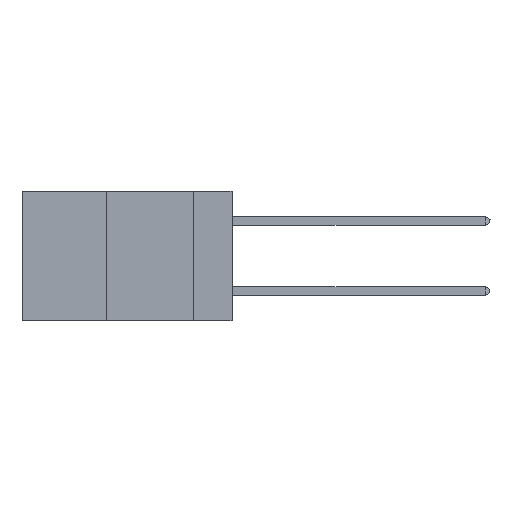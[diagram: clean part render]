
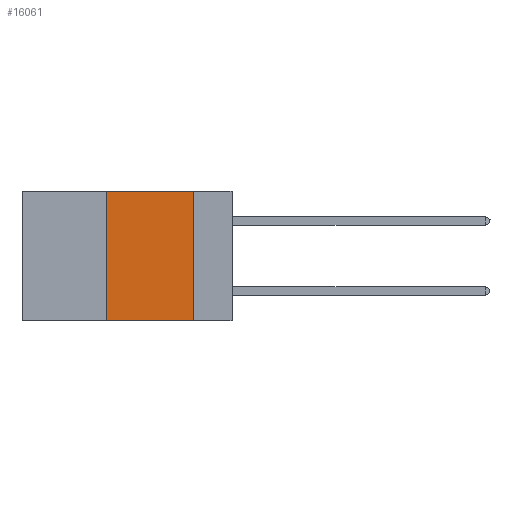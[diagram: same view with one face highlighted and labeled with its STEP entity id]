
A CAD part, left-side view. The second image highlights one B-rep face of the part: STEP entity #16061.
In plain terms, the highlighted planar face has unit normal (-1, 0, 0).
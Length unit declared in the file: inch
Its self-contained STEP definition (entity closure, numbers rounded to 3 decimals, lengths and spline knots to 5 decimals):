
#930 = DIRECTION ( 'NONE',  ( 0., -1., 0. ) ) ;
#1187 = DIRECTION ( 'NONE',  ( 0., 0., -1. ) ) ;
#3637 = LINE ( 'NONE', #10070, #5709 ) ;
#5500 = LINE ( 'NONE', #20741, #13701 ) ;
#5709 = VECTOR ( 'NONE', #46460, 39.37008 ) ;
#7206 = EDGE_CURVE ( 'NONE', #29236, #20243, #3637, .T. ) ;
#7396 = CARTESIAN_POINT ( 'NONE',  ( 0., 0.36, -0.37 ) ) ;
#7624 = ORIENTED_EDGE ( 'NONE', *, *, #7871, .T. ) ;
#7871 = EDGE_CURVE ( 'NONE', #9063, #38264, #19036, .T. ) ;
#8806 = CARTESIAN_POINT ( 'NONE',  ( 0., 0.6, 0. ) ) ;
#9063 = VERTEX_POINT ( 'NONE', #7396 ) ;
#10070 = CARTESIAN_POINT ( 'NONE',  ( 0., 0.6, 0. ) ) ;
#11123 = CARTESIAN_POINT ( 'NONE',  ( 0., 0.36, 0. ) ) ;
#11302 = CARTESIAN_POINT ( 'NONE',  ( 0., 0.11, 0. ) ) ;
#13701 = VECTOR ( 'NONE', #46193, 39.37008 ) ;
#15237 = CARTESIAN_POINT ( 'NONE',  ( 0., 0.11, -0.37 ) ) ;
#16061 = ADVANCED_FACE ( 'NONE', ( #23095 ), #33820, .F. ) ;
#16308 = EDGE_LOOP ( 'NONE', ( #23494, #27077, #42370, #7624 ) ) ;
#18735 = LINE ( 'NONE', #11123, #39338 ) ;
#18973 = DIRECTION ( 'NONE',  ( 0., 0., 1. ) ) ;
#19036 = LINE ( 'NONE', #33562, #39987 ) ;
#20243 = VERTEX_POINT ( 'NONE', #11302 ) ;
#20741 = CARTESIAN_POINT ( 'NONE',  ( 0., 0.11, 0. ) ) ;
#23095 = FACE_OUTER_BOUND ( 'NONE', #16308, .T. ) ;
#23328 = DIRECTION ( 'NONE',  ( 1., 0., 0. ) ) ;
#23494 = ORIENTED_EDGE ( 'NONE', *, *, #32778, .F. ) ;
#27077 = ORIENTED_EDGE ( 'NONE', *, *, #7206, .F. ) ;
#29236 = VERTEX_POINT ( 'NONE', #36227 ) ;
#31280 = AXIS2_PLACEMENT_3D ( 'NONE', #8806, #23328, #1187 ) ;
#32778 = EDGE_CURVE ( 'NONE', #20243, #38264, #5500, .T. ) ;
#33562 = CARTESIAN_POINT ( 'NONE',  ( 0., 0.6, -0.37 ) ) ;
#33820 = PLANE ( 'NONE',  #31280 ) ;
#36227 = CARTESIAN_POINT ( 'NONE',  ( 0., 0.36, 0. ) ) ;
#38264 = VERTEX_POINT ( 'NONE', #15237 ) ;
#39338 = VECTOR ( 'NONE', #18973, 39.37008 ) ;
#39987 = VECTOR ( 'NONE', #930, 39.37008 ) ;
#42370 = ORIENTED_EDGE ( 'NONE', *, *, #44447, .F. ) ;
#44447 = EDGE_CURVE ( 'NONE', #9063, #29236, #18735, .T. ) ;
#46193 = DIRECTION ( 'NONE',  ( 0., 0., -1. ) ) ;
#46460 = DIRECTION ( 'NONE',  ( 0., -1., 0. ) ) ;
